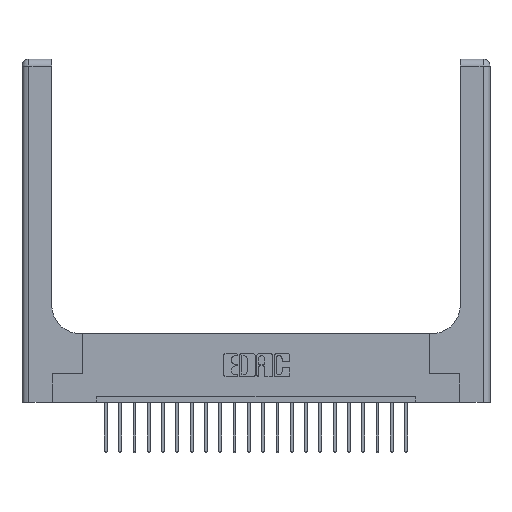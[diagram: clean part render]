
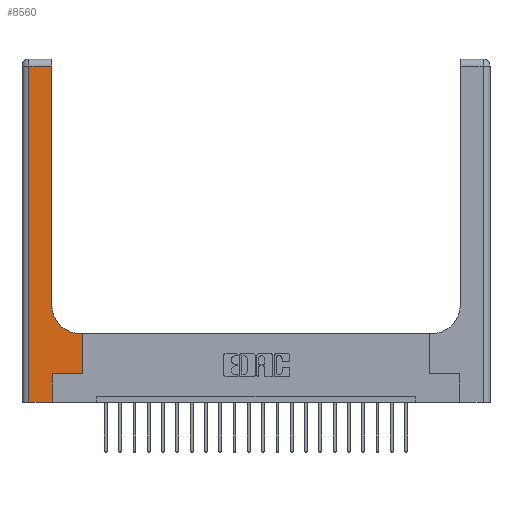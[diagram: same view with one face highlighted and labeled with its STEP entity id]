
A CAD part, top view. The second image highlights one B-rep face of the part: STEP entity #8560.
In plain terms, the highlighted planar face has unit normal (0, 0, 1).
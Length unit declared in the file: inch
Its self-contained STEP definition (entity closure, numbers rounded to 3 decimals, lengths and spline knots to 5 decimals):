
#4 = ORIENTED_EDGE ( 'NONE', *, *, #19269, .T. ) ;
#93 = VECTOR ( 'NONE', #10273, 39.37008 ) ;
#165 = VERTEX_POINT ( 'NONE', #21066 ) ;
#490 = CARTESIAN_POINT ( 'NONE',  ( 0.265, 0.25, 0.37 ) ) ;
#843 = ORIENTED_EDGE ( 'NONE', *, *, #9725, .T. ) ;
#1845 = ORIENTED_EDGE ( 'NONE', *, *, #20054, .T. ) ;
#1892 = ORIENTED_EDGE ( 'NONE', *, *, #3308, .T. ) ;
#2223 = VERTEX_POINT ( 'NONE', #17961 ) ;
#3308 = EDGE_CURVE ( 'NONE', #8434, #21158, #8675, .T. ) ;
#3787 = CARTESIAN_POINT ( 'NONE',  ( 0.265, 0., 0.37 ) ) ;
#3886 = CARTESIAN_POINT ( 'NONE',  ( 0.26, 2.94, 0.37 ) ) ;
#4432 = DIRECTION ( 'NONE',  ( 0., 0., -1. ) ) ;
#4496 = CARTESIAN_POINT ( 'NONE',  ( 0.528, 0.25, 0.37 ) ) ;
#4695 = LINE ( 'NONE', #15822, #13334 ) ;
#4827 = CARTESIAN_POINT ( 'NONE',  ( 0.26, 3., 0.37 ) ) ;
#4831 = ORIENTED_EDGE ( 'NONE', *, *, #9490, .T. ) ;
#5017 = DIRECTION ( 'NONE',  ( 0., 1., 0. ) ) ;
#5239 = VECTOR ( 'NONE', #5017, 39.37008 ) ;
#6843 = CIRCLE ( 'NONE', #12850, 0.25 ) ;
#7516 = DIRECTION ( 'NONE',  ( 1., 0., 0. ) ) ;
#7590 = CARTESIAN_POINT ( 'NONE',  ( 0.51, 0.85, 0.37 ) ) ;
#8063 = ORIENTED_EDGE ( 'NONE', *, *, #18250, .T. ) ;
#8434 = VERTEX_POINT ( 'NONE', #9269 ) ;
#8560 = ADVANCED_FACE ( 'NONE', ( #16528 ), #19350, .F. ) ;
#8675 = LINE ( 'NONE', #17892, #9449 ) ;
#8723 = VERTEX_POINT ( 'NONE', #16796 ) ;
#9269 = CARTESIAN_POINT ( 'NONE',  ( 0.06, 0., 0.37 ) ) ;
#9449 = VECTOR ( 'NONE', #16215, 39.37008 ) ;
#9490 = EDGE_CURVE ( 'NONE', #9577, #165, #10539, .T. ) ;
#9577 = VERTEX_POINT ( 'NONE', #3886 ) ;
#9600 = EDGE_CURVE ( 'NONE', #17441, #21312, #14130, .T. ) ;
#9725 = EDGE_CURVE ( 'NONE', #2223, #8723, #6843, .T. ) ;
#10127 = DIRECTION ( 'NONE',  ( 0., 1., 0. ) ) ;
#10153 = ORIENTED_EDGE ( 'NONE', *, *, #9600, .T. ) ;
#10273 = DIRECTION ( 'NONE',  ( -1., 0., 0. ) ) ;
#10529 = LINE ( 'NONE', #20068, #5239 ) ;
#10539 = LINE ( 'NONE', #11869, #93 ) ;
#11319 = CARTESIAN_POINT ( 'NONE',  ( 0., 3., 0.37 ) ) ;
#11869 = CARTESIAN_POINT ( 'NONE',  ( 0., 2.94, 0.37 ) ) ;
#11939 = DIRECTION ( 'NONE',  ( 1., 0., 0. ) ) ;
#12850 = AXIS2_PLACEMENT_3D ( 'NONE', #7590, #17485, #7516 ) ;
#13334 = VECTOR ( 'NONE', #17467, 39.37008 ) ;
#13607 = VECTOR ( 'NONE', #14393, 39.37008 ) ;
#13651 = EDGE_LOOP ( 'NONE', ( #1845, #4831, #4, #1892, #19509, #10153, #8063, #17566, #843 ) ) ;
#13964 = LINE ( 'NONE', #18716, #16066 ) ;
#14091 = CARTESIAN_POINT ( 'NONE',  ( 0.265, 0.25, 0.37 ) ) ;
#14130 = LINE ( 'NONE', #490, #18035 ) ;
#14393 = DIRECTION ( 'NONE',  ( -1., 0., 0. ) ) ;
#14400 = LINE ( 'NONE', #4827, #16476 ) ;
#15822 = CARTESIAN_POINT ( 'NONE',  ( 0.06, 3., 0.37 ) ) ;
#16024 = EDGE_CURVE ( 'NONE', #21158, #17441, #13964, .T. ) ;
#16066 = VECTOR ( 'NONE', #20204, 39.37008 ) ;
#16097 = DIRECTION ( 'NONE',  ( -1., 0., 0. ) ) ;
#16215 = DIRECTION ( 'NONE',  ( 1., 0., 0. ) ) ;
#16476 = VECTOR ( 'NONE', #10127, 39.37008 ) ;
#16528 = FACE_OUTER_BOUND ( 'NONE', #13651, .T. ) ;
#16796 = CARTESIAN_POINT ( 'NONE',  ( 0.26, 0.85, 0.37 ) ) ;
#17441 = VERTEX_POINT ( 'NONE', #14091 ) ;
#17467 = DIRECTION ( 'NONE',  ( 0., -1., 0. ) ) ;
#17485 = DIRECTION ( 'NONE',  ( 0., 0., -1. ) ) ;
#17566 = ORIENTED_EDGE ( 'NONE', *, *, #20433, .T. ) ;
#17776 = CARTESIAN_POINT ( 'NONE',  ( 0.528, 0.6, 0.37 ) ) ;
#17892 = CARTESIAN_POINT ( 'NONE',  ( 0., 0., 0.37 ) ) ;
#17961 = CARTESIAN_POINT ( 'NONE',  ( 0.51, 0.6, 0.37 ) ) ;
#18024 = LINE ( 'NONE', #19551, #13607 ) ;
#18035 = VECTOR ( 'NONE', #11939, 39.37008 ) ;
#18250 = EDGE_CURVE ( 'NONE', #21312, #20631, #10529, .T. ) ;
#18716 = CARTESIAN_POINT ( 'NONE',  ( 0.265, 0., 0.37 ) ) ;
#18948 = AXIS2_PLACEMENT_3D ( 'NONE', #11319, #4432, #16097 ) ;
#19269 = EDGE_CURVE ( 'NONE', #165, #8434, #4695, .T. ) ;
#19350 = PLANE ( 'NONE',  #18948 ) ;
#19509 = ORIENTED_EDGE ( 'NONE', *, *, #16024, .T. ) ;
#19551 = CARTESIAN_POINT ( 'NONE',  ( 0.26, 0.6, 0.37 ) ) ;
#20054 = EDGE_CURVE ( 'NONE', #8723, #9577, #14400, .T. ) ;
#20068 = CARTESIAN_POINT ( 'NONE',  ( 0.528, 0.25, 0.37 ) ) ;
#20204 = DIRECTION ( 'NONE',  ( 0., 1., 0. ) ) ;
#20433 = EDGE_CURVE ( 'NONE', #20631, #2223, #18024, .T. ) ;
#20631 = VERTEX_POINT ( 'NONE', #17776 ) ;
#21066 = CARTESIAN_POINT ( 'NONE',  ( 0.06, 2.94, 0.37 ) ) ;
#21158 = VERTEX_POINT ( 'NONE', #3787 ) ;
#21312 = VERTEX_POINT ( 'NONE', #4496 ) ;
